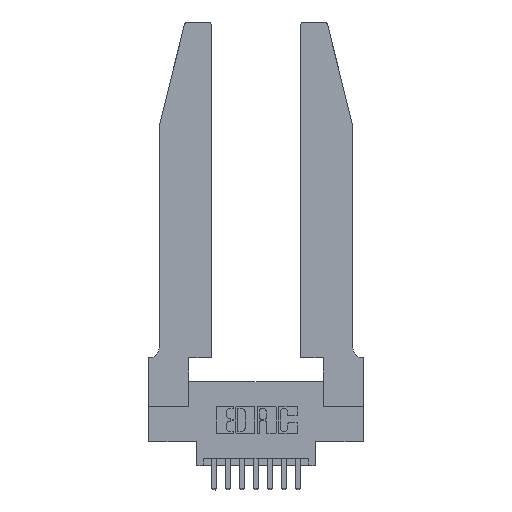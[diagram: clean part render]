
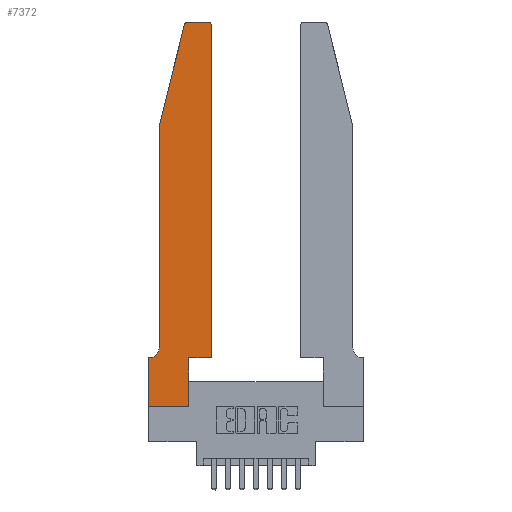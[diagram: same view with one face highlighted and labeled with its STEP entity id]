
A CAD part, top view. The second image highlights one B-rep face of the part: STEP entity #7372.
In plain terms, the highlighted planar face has unit normal (0, 0, 1).
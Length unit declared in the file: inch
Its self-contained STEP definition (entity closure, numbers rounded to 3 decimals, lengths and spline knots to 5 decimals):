
#70 = LINE ( 'NONE', #2637, #6830 ) ;
#100 = CIRCLE ( 'NONE', #5580, 0.07 ) ;
#292 = ORIENTED_EDGE ( 'NONE', *, *, #6726, .T. ) ;
#835 = LINE ( 'NONE', #1937, #7755 ) ;
#911 = CARTESIAN_POINT ( 'NONE',  ( 0.0055, 0.35, 0.37 ) ) ;
#1525 = VECTOR ( 'NONE', #13273, 39.37008 ) ;
#1643 = EDGE_CURVE ( 'NONE', #14787, #12640, #70, .T. ) ;
#1937 = CARTESIAN_POINT ( 'NONE',  ( 0., 0., 0.37 ) ) ;
#2145 = DIRECTION ( 'NONE',  ( -1., 0., 0. ) ) ;
#2487 = EDGE_CURVE ( 'NONE', #14289, #14787, #8835, .T. ) ;
#2537 = VERTEX_POINT ( 'NONE', #9928 ) ;
#2541 = VECTOR ( 'NONE', #2145, 39.37008 ) ;
#2637 = CARTESIAN_POINT ( 'NONE',  ( 0.0755, 2., 0.37 ) ) ;
#2805 = ORIENTED_EDGE ( 'NONE', *, *, #5799, .T. ) ;
#2859 = DIRECTION ( 'NONE',  ( 0., 0., 1. ) ) ;
#2910 = ORIENTED_EDGE ( 'NONE', *, *, #15144, .T. ) ;
#3069 = VECTOR ( 'NONE', #13577, 39.37008 ) ;
#3500 = EDGE_CURVE ( 'NONE', #11086, #7527, #10245, .T. ) ;
#3512 = ORIENTED_EDGE ( 'NONE', *, *, #3500, .T. ) ;
#3755 = CARTESIAN_POINT ( 'NONE',  ( 0.0755, 0.35, 0.37 ) ) ;
#4000 = CARTESIAN_POINT ( 'NONE',  ( 0.284, 2.75, 0.37 ) ) ;
#4396 = CARTESIAN_POINT ( 'NONE',  ( 0.0055, 0.42, 0.37 ) ) ;
#4432 = ORIENTED_EDGE ( 'NONE', *, *, #7958, .T. ) ;
#4592 = VERTEX_POINT ( 'NONE', #13900 ) ;
#4615 = AXIS2_PLACEMENT_3D ( 'NONE', #8414, #14367, #9454 ) ;
#4940 = EDGE_CURVE ( 'NONE', #12640, #11207, #100, .T. ) ;
#4959 = CIRCLE ( 'NONE', #12781, 0.03 ) ;
#5175 = VECTOR ( 'NONE', #10370, 39.37008 ) ;
#5188 = DIRECTION ( 'NONE',  ( 1., 0., 0. ) ) ;
#5387 = CARTESIAN_POINT ( 'NONE',  ( 0.4205, 2.75, 0.37 ) ) ;
#5439 = ORIENTED_EDGE ( 'NONE', *, *, #1643, .T. ) ;
#5580 = AXIS2_PLACEMENT_3D ( 'NONE', #4396, #9145, #8057 ) ;
#5698 = CARTESIAN_POINT ( 'NONE',  ( 0.4205, 2.72, 0.37 ) ) ;
#5700 = CARTESIAN_POINT ( 'NONE',  ( 0., 0., 0.37 ) ) ;
#5799 = EDGE_CURVE ( 'NONE', #4592, #6578, #835, .T. ) ;
#6058 = CARTESIAN_POINT ( 'NONE',  ( 0.2865, 0.35, 0.37 ) ) ;
#6382 = CARTESIAN_POINT ( 'NONE',  ( 0.2865, 0., 0.37 ) ) ;
#6394 = DIRECTION ( 'NONE',  ( 1., 0., 0. ) ) ;
#6578 = VERTEX_POINT ( 'NONE', #6382 ) ;
#6686 = ORIENTED_EDGE ( 'NONE', *, *, #2487, .T. ) ;
#6726 = EDGE_CURVE ( 'NONE', #11511, #4592, #13818, .T. ) ;
#6830 = VECTOR ( 'NONE', #14652, 39.37008 ) ;
#6941 = CARTESIAN_POINT ( 'NONE',  ( 0.4505, 0.35, 0.37 ) ) ;
#7372 = ADVANCED_FACE ( 'NONE', ( #12723 ), #14214, .T. ) ;
#7410 = CARTESIAN_POINT ( 'NONE',  ( 0.0755, 0.42, 0.37 ) ) ;
#7527 = VERTEX_POINT ( 'NONE', #4000 ) ;
#7755 = VECTOR ( 'NONE', #5188, 39.37008 ) ;
#7806 = CARTESIAN_POINT ( 'NONE',  ( 0.0755, 2., 0.37 ) ) ;
#7846 = DIRECTION ( 'NONE',  ( 1., 0., 0. ) ) ;
#7958 = EDGE_CURVE ( 'NONE', #11909, #2537, #10115, .T. ) ;
#8057 = DIRECTION ( 'NONE',  ( -1., 0., 0. ) ) ;
#8074 = DIRECTION ( 'NONE',  ( 0., 0., 1. ) ) ;
#8217 = CARTESIAN_POINT ( 'NONE',  ( 0.2865, 0.35, 0.37 ) ) ;
#8414 = CARTESIAN_POINT ( 'NONE',  ( 0., 0.35, 0.37 ) ) ;
#8453 = ORIENTED_EDGE ( 'NONE', *, *, #9671, .T. ) ;
#8619 = EDGE_CURVE ( 'NONE', #7527, #14289, #4959, .T. ) ;
#8835 = LINE ( 'NONE', #9738, #1525 ) ;
#9145 = DIRECTION ( 'NONE',  ( 0., 0., -1. ) ) ;
#9454 = DIRECTION ( 'NONE',  ( 1., 0., 0. ) ) ;
#9502 = LINE ( 'NONE', #3755, #14891 ) ;
#9671 = EDGE_CURVE ( 'NONE', #11207, #11511, #9502, .T. ) ;
#9738 = CARTESIAN_POINT ( 'NONE',  ( 0.0755, 2., 0.37 ) ) ;
#9768 = CIRCLE ( 'NONE', #13290, 0.03 ) ;
#9776 = ORIENTED_EDGE ( 'NONE', *, *, #4940, .T. ) ;
#9928 = CARTESIAN_POINT ( 'NONE',  ( 0.4505, 0.35, 0.37 ) ) ;
#10115 = LINE ( 'NONE', #13783, #14563 ) ;
#10245 = LINE ( 'NONE', #15029, #2541 ) ;
#10315 = CARTESIAN_POINT ( 'NONE',  ( 0.25487, 2.72718, 0.37 ) ) ;
#10363 = VERTEX_POINT ( 'NONE', #13445 ) ;
#10370 = DIRECTION ( 'NONE',  ( 0., -1., 0. ) ) ;
#10505 = LINE ( 'NONE', #6058, #15133 ) ;
#11086 = VERTEX_POINT ( 'NONE', #5387 ) ;
#11207 = VERTEX_POINT ( 'NONE', #911 ) ;
#11238 = ORIENTED_EDGE ( 'NONE', *, *, #14182, .T. ) ;
#11452 = DIRECTION ( 'NONE',  ( 1., 0., 0. ) ) ;
#11511 = VERTEX_POINT ( 'NONE', #14381 ) ;
#11677 = EDGE_CURVE ( 'NONE', #2537, #10363, #11872, .T. ) ;
#11872 = LINE ( 'NONE', #6941, #3069 ) ;
#11909 = VERTEX_POINT ( 'NONE', #8217 ) ;
#12640 = VERTEX_POINT ( 'NONE', #7410 ) ;
#12723 = FACE_OUTER_BOUND ( 'NONE', #13630, .T. ) ;
#12781 = AXIS2_PLACEMENT_3D ( 'NONE', #13217, #2859, #6394 ) ;
#12942 = DIRECTION ( 'NONE',  ( 0., 1., 0. ) ) ;
#13217 = CARTESIAN_POINT ( 'NONE',  ( 0.284, 2.72, 0.37 ) ) ;
#13273 = DIRECTION ( 'NONE',  ( -0.239, -0.971, 0. ) ) ;
#13290 = AXIS2_PLACEMENT_3D ( 'NONE', #5698, #8074, #11452 ) ;
#13445 = CARTESIAN_POINT ( 'NONE',  ( 0.4505, 2.72, 0.37 ) ) ;
#13577 = DIRECTION ( 'NONE',  ( 0., 1., 0. ) ) ;
#13630 = EDGE_LOOP ( 'NONE', ( #3512, #13736, #6686, #5439, #9776, #8453, #292, #2805, #2910, #4432, #13935, #11238 ) ) ;
#13736 = ORIENTED_EDGE ( 'NONE', *, *, #8619, .T. ) ;
#13783 = CARTESIAN_POINT ( 'NONE',  ( 0.4505, 0.35, 0.37 ) ) ;
#13818 = LINE ( 'NONE', #5700, #5175 ) ;
#13900 = CARTESIAN_POINT ( 'NONE',  ( 0., 0., 0.37 ) ) ;
#13935 = ORIENTED_EDGE ( 'NONE', *, *, #11677, .T. ) ;
#14182 = EDGE_CURVE ( 'NONE', #10363, #11086, #9768, .T. ) ;
#14214 = PLANE ( 'NONE',  #4615 ) ;
#14289 = VERTEX_POINT ( 'NONE', #10315 ) ;
#14367 = DIRECTION ( 'NONE',  ( 0., 0., 1. ) ) ;
#14381 = CARTESIAN_POINT ( 'NONE',  ( 0., 0.35, 0.37 ) ) ;
#14401 = DIRECTION ( 'NONE',  ( -1., 0., 0. ) ) ;
#14563 = VECTOR ( 'NONE', #7846, 39.37008 ) ;
#14652 = DIRECTION ( 'NONE',  ( 0., -1., 0. ) ) ;
#14787 = VERTEX_POINT ( 'NONE', #7806 ) ;
#14891 = VECTOR ( 'NONE', #14401, 39.37008 ) ;
#15029 = CARTESIAN_POINT ( 'NONE',  ( 0.2605, 2.75, 0.37 ) ) ;
#15133 = VECTOR ( 'NONE', #12942, 39.37008 ) ;
#15144 = EDGE_CURVE ( 'NONE', #6578, #11909, #10505, .T. ) ;
